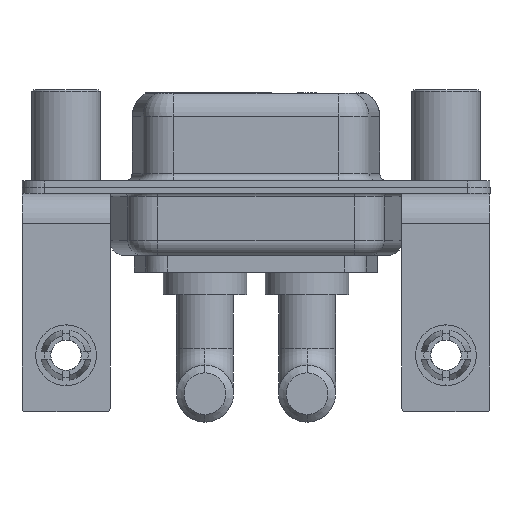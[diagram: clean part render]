
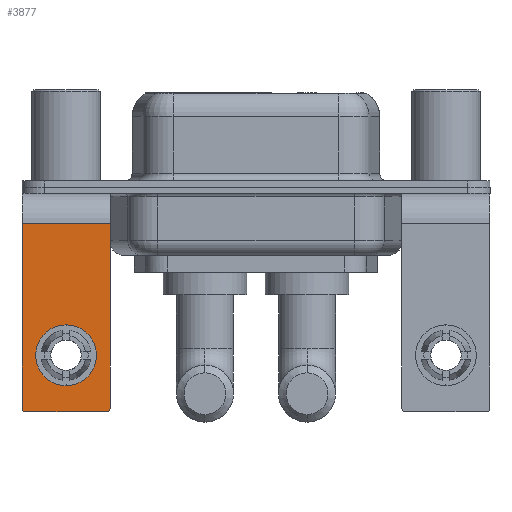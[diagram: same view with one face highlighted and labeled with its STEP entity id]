
A CAD part, front view. The second image highlights one B-rep face of the part: STEP entity #3877.
In plain terms, the highlighted planar face has unit normal (0, -1, 0).
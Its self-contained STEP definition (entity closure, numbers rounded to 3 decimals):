
#78 = VERTEX_POINT ( 'NONE', #5016 ) ;
#234 = EDGE_CURVE ( 'NONE', #2490, #7900, #16105, .T. ) ;
#384 = EDGE_CURVE ( 'NONE', #2856, #16089, #5103, .T. ) ;
#977 = DIRECTION ( 'NONE',  ( 0., -1., 0. ) ) ;
#1061 = ORIENTED_EDGE ( 'NONE', *, *, #5054, .T. ) ;
#1151 = DIRECTION ( 'NONE',  ( 0., 0., 1. ) ) ;
#1248 = VERTEX_POINT ( 'NONE', #12286 ) ;
#1536 = EDGE_CURVE ( 'NONE', #1248, #78, #6267, .T. ) ;
#1648 = DIRECTION ( 'NONE',  ( 0., 0., -1. ) ) ;
#1782 = VECTOR ( 'NONE', #17290, 1000. ) ;
#1950 = CIRCLE ( 'NONE', #9026, 0.25 ) ;
#2198 = ORIENTED_EDGE ( 'NONE', *, *, #11092, .F. ) ;
#2490 = VERTEX_POINT ( 'NONE', #11210 ) ;
#2523 = CARTESIAN_POINT ( 'NONE',  ( -2.9, -6.25, -2.4 ) ) ;
#2756 = DIRECTION ( 'NONE',  ( 0., 1., 0. ) ) ;
#2765 = AXIS2_PLACEMENT_3D ( 'NONE', #11978, #15946, #5169 ) ;
#2856 = VERTEX_POINT ( 'NONE', #11930 ) ;
#2943 = ORIENTED_EDGE ( 'NONE', *, *, #5421, .T. ) ;
#3277 = AXIS2_PLACEMENT_3D ( 'NONE', #4018, #2756, #10977 ) ;
#3877 = ADVANCED_FACE ( 'NONE', ( #9230, #7659 ), #9147, .F. ) ;
#4018 = CARTESIAN_POINT ( 'NONE',  ( 0., -6.25, -11.07 ) ) ;
#4374 = DIRECTION ( 'NONE',  ( 0., 1., 0. ) ) ;
#4794 = VERTEX_POINT ( 'NONE', #6587 ) ;
#5012 = CARTESIAN_POINT ( 'NONE',  ( 0., -6.25, -13.07 ) ) ;
#5016 = CARTESIAN_POINT ( 'NONE',  ( -2.9, -6.25, -2.4 ) ) ;
#5054 = EDGE_CURVE ( 'NONE', #16089, #2856, #10897, .T. ) ;
#5103 = CIRCLE ( 'NONE', #12159, 2. ) ;
#5169 = DIRECTION ( 'NONE',  ( 0., 0., 1. ) ) ;
#5421 = EDGE_CURVE ( 'NONE', #4794, #8251, #1950, .T. ) ;
#6045 = VECTOR ( 'NONE', #10768, 1000. ) ;
#6059 = CARTESIAN_POINT ( 'NONE',  ( 0., -6.25, -11.07 ) ) ;
#6267 = LINE ( 'NONE', #13264, #8860 ) ;
#6587 = CARTESIAN_POINT ( 'NONE',  ( -2.9, -6.25, -14.55 ) ) ;
#6964 = ORIENTED_EDGE ( 'NONE', *, *, #7471, .F. ) ;
#7038 = DIRECTION ( 'NONE',  ( 0., -1., 0. ) ) ;
#7471 = EDGE_CURVE ( 'NONE', #2490, #8251, #8044, .T. ) ;
#7659 = FACE_OUTER_BOUND ( 'NONE', #12308, .T. ) ;
#7725 = CARTESIAN_POINT ( 'NONE',  ( -2.65, -6.25, -14.55 ) ) ;
#7875 = EDGE_CURVE ( 'NONE', #78, #4794, #16145, .T. ) ;
#7900 = VERTEX_POINT ( 'NONE', #10833 ) ;
#8044 = LINE ( 'NONE', #9529, #6045 ) ;
#8251 = VERTEX_POINT ( 'NONE', #9642 ) ;
#8342 = VECTOR ( 'NONE', #1648, 1000. ) ;
#8860 = VECTOR ( 'NONE', #15887, 1000. ) ;
#9026 = AXIS2_PLACEMENT_3D ( 'NONE', #7725, #977, #1151 ) ;
#9147 = PLANE ( 'NONE',  #2765 ) ;
#9230 = FACE_BOUND ( 'NONE', #13075, .T. ) ;
#9330 = AXIS2_PLACEMENT_3D ( 'NONE', #16211, #7038, #13681 ) ;
#9363 = ORIENTED_EDGE ( 'NONE', *, *, #7875, .T. ) ;
#9444 = CARTESIAN_POINT ( 'NONE',  ( 2.9, -6.25, -2.4 ) ) ;
#9529 = CARTESIAN_POINT ( 'NONE',  ( 2.9, -6.25, -14.8 ) ) ;
#9530 = LINE ( 'NONE', #9444, #8342 ) ;
#9642 = CARTESIAN_POINT ( 'NONE',  ( -2.65, -6.25, -14.8 ) ) ;
#10241 = ORIENTED_EDGE ( 'NONE', *, *, #234, .T. ) ;
#10768 = DIRECTION ( 'NONE',  ( -1., 0., 0. ) ) ;
#10833 = CARTESIAN_POINT ( 'NONE',  ( 2.9, -6.25, -14.55 ) ) ;
#10897 = CIRCLE ( 'NONE', #3277, 2. ) ;
#10977 = DIRECTION ( 'NONE',  ( 0., 0., 1. ) ) ;
#11092 = EDGE_CURVE ( 'NONE', #1248, #7900, #9530, .T. ) ;
#11210 = CARTESIAN_POINT ( 'NONE',  ( 2.65, -6.25, -14.8 ) ) ;
#11445 = DIRECTION ( 'NONE',  ( 0., 0., 1. ) ) ;
#11930 = CARTESIAN_POINT ( 'NONE',  ( 0., -6.25, -9.07 ) ) ;
#11978 = CARTESIAN_POINT ( 'NONE',  ( 2.9, -6.25, -2.4 ) ) ;
#12159 = AXIS2_PLACEMENT_3D ( 'NONE', #6059, #4374, #11445 ) ;
#12286 = CARTESIAN_POINT ( 'NONE',  ( 2.9, -6.25, -2.4 ) ) ;
#12308 = EDGE_LOOP ( 'NONE', ( #9363, #2943, #6964, #10241, #2198, #13922 ) ) ;
#13075 = EDGE_LOOP ( 'NONE', ( #1061, #13306 ) ) ;
#13264 = CARTESIAN_POINT ( 'NONE',  ( 2.9, -6.25, -2.4 ) ) ;
#13306 = ORIENTED_EDGE ( 'NONE', *, *, #384, .T. ) ;
#13681 = DIRECTION ( 'NONE',  ( 0., 0., 1. ) ) ;
#13922 = ORIENTED_EDGE ( 'NONE', *, *, #1536, .T. ) ;
#15887 = DIRECTION ( 'NONE',  ( -1., 0., 0. ) ) ;
#15946 = DIRECTION ( 'NONE',  ( 0., 1., 0. ) ) ;
#16089 = VERTEX_POINT ( 'NONE', #5012 ) ;
#16105 = CIRCLE ( 'NONE', #9330, 0.25 ) ;
#16145 = LINE ( 'NONE', #2523, #1782 ) ;
#16211 = CARTESIAN_POINT ( 'NONE',  ( 2.65, -6.25, -14.55 ) ) ;
#17290 = DIRECTION ( 'NONE',  ( 0., 0., -1. ) ) ;
